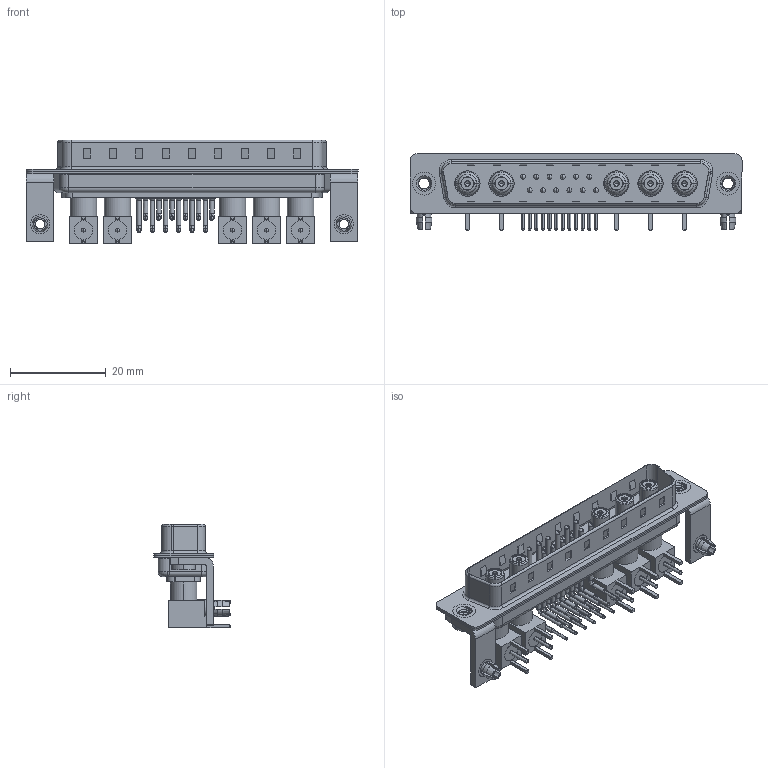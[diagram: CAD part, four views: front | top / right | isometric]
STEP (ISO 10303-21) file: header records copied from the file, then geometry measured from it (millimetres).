
FILE_DESCRIPTION (( 'STEP AP203' ), '1' );
FILE_NAME ('629-17W5640-7NB.STEP', '2022-05-16T00:47:57', ( '' ), ( '' ), 'SwSTEP 2.0', 'SolidWorks 2020', '' );
FILE_SCHEMA (( 'CONFIG_CONTROL_DESIGN' ));
Length unit declared in the file: millimetre
Products named in the file (21): RA Back Shell; Locking Collar; Co-Ax Jack Assy_RA; Insulator RA Pin; Insulator Socket 2; Insulator Socket; 629Combo Board Lock; 629Combo Shell Rear_37 Contacts; 629Combo Threaded Rivet_2; Socket_RA; 629Combo Shell Front_37 Contacts; 629Combo Housing_17W5; 629Combo Stabilizer Bracket; 629-17W5640-7NB; 629Combo Contact Row 1; 629Combo Contact Row 2; Co-Ax Jack_RA PC Tail
Assembly tree (61 placements, depth 3):
  629-17W5640-7NB
    629Combo Housing_17W5
    629Combo Shell Rear_37 Contacts
    629Combo Shell Front_37 Contacts
    629Combo Threaded Rivet_2  x2
    629Combo Stabilizer Bracket  x2
    629Combo Board Lock  x2
    Co-Ax Jack Assy_RA
      Co-Ax Jack_RA PC Tail
      Insulator Socket
      Insulator Socket 2
      Locking Collar
      Socket_RA
      RA Back Shell
      Insulator RA Pin
    Co-Ax Jack Assy_RA
      Co-Ax Jack_RA PC Tail
      Insulator Socket
      Insulator Socket 2
      Locking Collar
      Socket_RA
      RA Back Shell
      Insulator RA Pin
    Co-Ax Jack Assy_RA
      Co-Ax Jack_RA PC Tail
      Insulator Socket
      Insulator Socket 2
      Locking Collar
      Socket_RA
      RA Back Shell
      Insulator RA Pin
    Co-Ax Jack Assy_RA
      Co-Ax Jack_RA PC Tail
      Insulator Socket
      Insulator Socket 2
      Locking Collar
      Socket_RA
      RA Back Shell
      Insulator RA Pin
    Co-Ax Jack Assy_RA
      Co-Ax Jack_RA PC Tail
      Insulator Socket
      Insulator Socket 2
      Locking Collar
      Socket_RA
      RA Back Shell
      Insulator RA Pin
    629Combo Contact Row 1  x6
    629Combo Contact Row 2  x6
Bounding box: 69.4 x 16 x 21.71 mm (x, y, z)
Volume: 5639.1 mm3; surface area: 15063.7 mm2
Topology: 56 solids, 56 shells, 2632 faces, 6886 edges, 4411 vertices
Faces by surface type: plane 1324, cylinder 964, cone 171, bspline 83, torus 80, sphere 10
Entity records: 33308 total; most frequent: CARTESIAN_POINT 6790, DIRECTION 5074, ORIENTED_EDGE 4674, EDGE_CURVE 2337, AXIS2_PLACEMENT_3D 1836, VERTEX_POINT 1505, LINE 1402, VECTOR 1402
